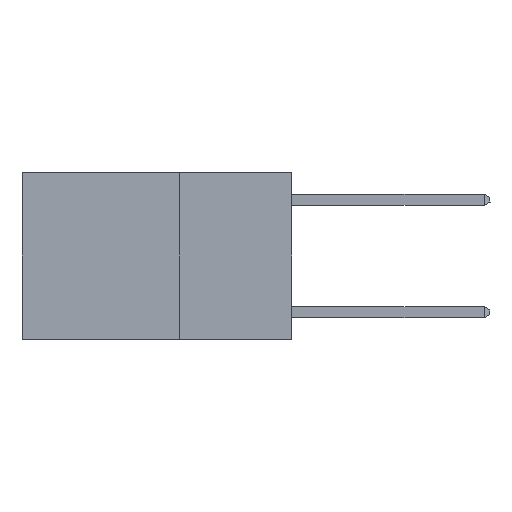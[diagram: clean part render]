
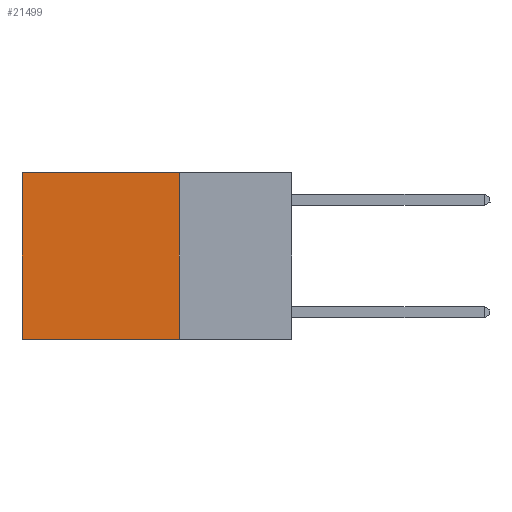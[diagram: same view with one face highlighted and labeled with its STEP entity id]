
A CAD part, left-side view. The second image highlights one B-rep face of the part: STEP entity #21499.
In plain terms, the highlighted planar face has unit normal (-1, 0, 0).
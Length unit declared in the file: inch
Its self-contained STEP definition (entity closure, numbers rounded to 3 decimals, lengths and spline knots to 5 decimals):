
#1175 = VECTOR ( 'NONE', #7551, 39.37008 ) ;
#2142 = VERTEX_POINT ( 'NONE', #12577 ) ;
#2571 = ORIENTED_EDGE ( 'NONE', *, *, #22078, .F. ) ;
#4138 = EDGE_CURVE ( 'NONE', #17461, #16575, #6245, .T. ) ;
#4852 = EDGE_LOOP ( 'NONE', ( #22548, #20945, #2571, #8983 ) ) ;
#5859 = PLANE ( 'NONE',  #9056 ) ;
#6245 = LINE ( 'NONE', #14672, #23126 ) ;
#7551 = DIRECTION ( 'NONE',  ( 0., 0., -1. ) ) ;
#7956 = FACE_OUTER_BOUND ( 'NONE', #4852, .T. ) ;
#8291 = DIRECTION ( 'NONE',  ( 0., 0., -1. ) ) ;
#8905 = EDGE_CURVE ( 'NONE', #2142, #16575, #14165, .T. ) ;
#8983 = ORIENTED_EDGE ( 'NONE', *, *, #13598, .T. ) ;
#9056 = AXIS2_PLACEMENT_3D ( 'NONE', #20546, #18207, #20418 ) ;
#12577 = CARTESIAN_POINT ( 'NONE',  ( 0.2625, 0.6, 0. ) ) ;
#13598 = EDGE_CURVE ( 'NONE', #21055, #2142, #26422, .T. ) ;
#13880 = CARTESIAN_POINT ( 'NONE',  ( 0.2625, 0.6, 0. ) ) ;
#14165 = LINE ( 'NONE', #13880, #1175 ) ;
#14672 = CARTESIAN_POINT ( 'NONE',  ( 0.2625, 0.25, -0.37 ) ) ;
#15590 = CARTESIAN_POINT ( 'NONE',  ( 0.2625, 0.25, -0.37 ) ) ;
#16575 = VERTEX_POINT ( 'NONE', #19614 ) ;
#17461 = VERTEX_POINT ( 'NONE', #15590 ) ;
#17676 = VECTOR ( 'NONE', #20328, 39.37008 ) ;
#18207 = DIRECTION ( 'NONE',  ( 1., 0., 0. ) ) ;
#19614 = CARTESIAN_POINT ( 'NONE',  ( 0.2625, 0.6, -0.37 ) ) ;
#20328 = DIRECTION ( 'NONE',  ( 0., 1., 0. ) ) ;
#20418 = DIRECTION ( 'NONE',  ( 0., 0., -1. ) ) ;
#20546 = CARTESIAN_POINT ( 'NONE',  ( 0.2625, 0.25, 0. ) ) ;
#20891 = LINE ( 'NONE', #27254, #21464 ) ;
#20945 = ORIENTED_EDGE ( 'NONE', *, *, #4138, .F. ) ;
#21055 = VERTEX_POINT ( 'NONE', #23988 ) ;
#21464 = VECTOR ( 'NONE', #8291, 39.37008 ) ;
#21499 = ADVANCED_FACE ( 'NONE', ( #7956 ), #5859, .F. ) ;
#22078 = EDGE_CURVE ( 'NONE', #21055, #17461, #20891, .T. ) ;
#22548 = ORIENTED_EDGE ( 'NONE', *, *, #8905, .T. ) ;
#23124 = DIRECTION ( 'NONE',  ( 0., 1., 0. ) ) ;
#23126 = VECTOR ( 'NONE', #23124, 39.37008 ) ;
#23988 = CARTESIAN_POINT ( 'NONE',  ( 0.2625, 0.25, 0. ) ) ;
#26422 = LINE ( 'NONE', #26556, #17676 ) ;
#26556 = CARTESIAN_POINT ( 'NONE',  ( 0.2625, 0.25, 0. ) ) ;
#27254 = CARTESIAN_POINT ( 'NONE',  ( 0.2625, 0.25, 0. ) ) ;
